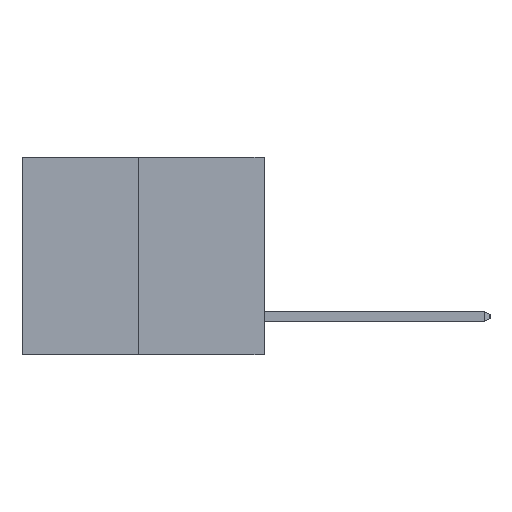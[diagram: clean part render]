
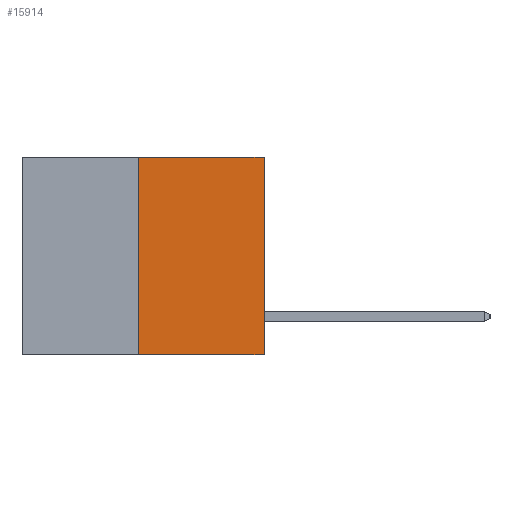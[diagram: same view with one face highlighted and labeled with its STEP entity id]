
A CAD part, left-side view. The second image highlights one B-rep face of the part: STEP entity #15914.
In plain terms, the highlighted planar face has unit normal (-1, 0, 0).
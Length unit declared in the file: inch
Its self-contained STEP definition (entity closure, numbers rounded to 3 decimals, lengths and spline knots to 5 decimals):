
#773 = EDGE_CURVE ( 'NONE', #14973, #6611, #5121, .T. ) ;
#2016 = DIRECTION ( 'NONE',  ( 0., -1., 0. ) ) ;
#2266 = VECTOR ( 'NONE', #2016, 39.37008 ) ;
#2724 = EDGE_CURVE ( 'NONE', #6611, #17098, #9687, .T. ) ;
#2944 = CARTESIAN_POINT ( 'NONE',  ( 0., 0.6, -0.49 ) ) ;
#3335 = DIRECTION ( 'NONE',  ( 0., 0., 1. ) ) ;
#3348 = DIRECTION ( 'NONE',  ( 0., 0., 1. ) ) ;
#3734 = LINE ( 'NONE', #7357, #2266 ) ;
#4248 = VECTOR ( 'NONE', #3335, 39.37008 ) ;
#4302 = DIRECTION ( 'NONE',  ( 0., -1., 0. ) ) ;
#5121 = LINE ( 'NONE', #2944, #6825 ) ;
#6091 = VECTOR ( 'NONE', #3348, 39.37008 ) ;
#6265 = CARTESIAN_POINT ( 'NONE',  ( 0., 0., -0.49 ) ) ;
#6611 = VERTEX_POINT ( 'NONE', #6265 ) ;
#6825 = VECTOR ( 'NONE', #4302, 39.37008 ) ;
#7357 = CARTESIAN_POINT ( 'NONE',  ( 0., 0.6, 0. ) ) ;
#7557 = EDGE_LOOP ( 'NONE', ( #9898, #14255, #12961, #12337 ) ) ;
#7768 = FACE_OUTER_BOUND ( 'NONE', #7557, .T. ) ;
#7817 = LINE ( 'NONE', #10014, #4248 ) ;
#7922 = VERTEX_POINT ( 'NONE', #14343 ) ;
#8057 = CARTESIAN_POINT ( 'NONE',  ( 0., 0., 0. ) ) ;
#8282 = CARTESIAN_POINT ( 'NONE',  ( 0., 0.6, 0. ) ) ;
#9687 = LINE ( 'NONE', #10502, #6091 ) ;
#9874 = AXIS2_PLACEMENT_3D ( 'NONE', #8282, #14712, #13436 ) ;
#9898 = ORIENTED_EDGE ( 'NONE', *, *, #11116, .F. ) ;
#10014 = CARTESIAN_POINT ( 'NONE',  ( 0., 0.312, -0.49 ) ) ;
#10502 = CARTESIAN_POINT ( 'NONE',  ( 0., 0., 0. ) ) ;
#11116 = EDGE_CURVE ( 'NONE', #14973, #7922, #7817, .T. ) ;
#12337 = ORIENTED_EDGE ( 'NONE', *, *, #16884, .F. ) ;
#12961 = ORIENTED_EDGE ( 'NONE', *, *, #2724, .T. ) ;
#13436 = DIRECTION ( 'NONE',  ( 0., 0., -1. ) ) ;
#14255 = ORIENTED_EDGE ( 'NONE', *, *, #773, .T. ) ;
#14343 = CARTESIAN_POINT ( 'NONE',  ( 0., 0.312, 0. ) ) ;
#14712 = DIRECTION ( 'NONE',  ( 1., 0., 0. ) ) ;
#14973 = VERTEX_POINT ( 'NONE', #16887 ) ;
#15914 = ADVANCED_FACE ( 'NONE', ( #7768 ), #16230, .F. ) ;
#16230 = PLANE ( 'NONE',  #9874 ) ;
#16884 = EDGE_CURVE ( 'NONE', #7922, #17098, #3734, .T. ) ;
#16887 = CARTESIAN_POINT ( 'NONE',  ( 0., 0.312, -0.49 ) ) ;
#17098 = VERTEX_POINT ( 'NONE', #8057 ) ;
